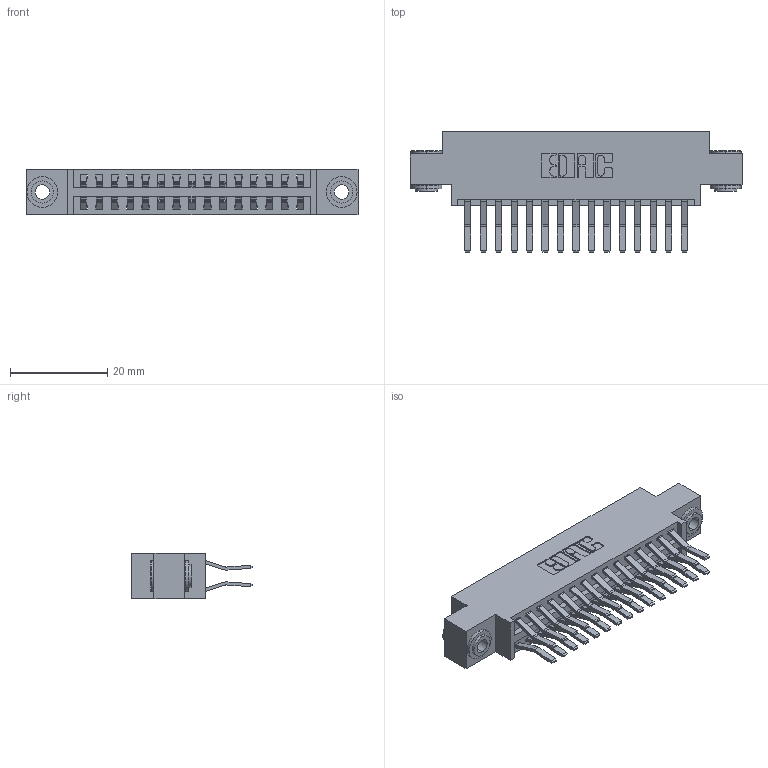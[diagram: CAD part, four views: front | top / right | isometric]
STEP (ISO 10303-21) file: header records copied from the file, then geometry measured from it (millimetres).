
FILE_DESCRIPTION (( 'STEP AP203' ), '1' );
FILE_NAME ('346-030-560-803.STEP', '2018-08-22T06:26:04', ( '' ), ( '' ), 'SwSTEP 2.0', 'SolidWorks 2016', '' );
FILE_SCHEMA (( 'CONFIG_CONTROL_DESIGN' ));
Length unit declared in the file: inch
Products named in the file (4): 346 Part_0.170 Offset - 0.156 Dia-TH; 345-292-001_560 Tail; 345-250-002_345-250-002-102; 346-030-560-803
Assembly tree (33 placements, depth 2):
  346-030-560-803
    346 Part_0.170 Offset - 0.156 Dia-TH
    345-292-001_560 Tail  x30
    345-250-002_345-250-002-102  x2
Bounding box: 68.2 x 24.78 x 9.4 mm (x, y, z)
Volume: 6502 mm3; surface area: 9431.4 mm2
Topology: 33 solids, 33 shells, 1784 faces, 5247 edges, 3454 vertices
Faces by surface type: plane 1140, cylinder 636, cone 8
Entity records: 14294 total; most frequent: CARTESIAN_POINT 2371, ORIENTED_EDGE 2298, DIRECTION 2175, EDGE_CURVE 1149, VECTOR 929, LINE 929, VERTEX_POINT 762, AXIS2_PLACEMENT_3D 623
